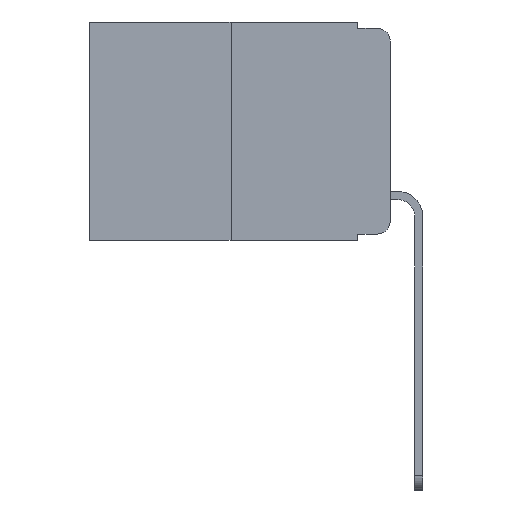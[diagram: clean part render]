
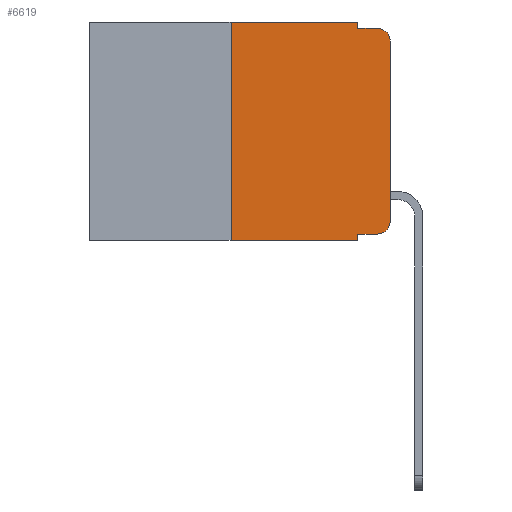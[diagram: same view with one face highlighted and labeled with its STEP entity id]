
A CAD part, left-side view. The second image highlights one B-rep face of the part: STEP entity #6619.
In plain terms, the highlighted planar face has unit normal (-1, 0, 0).
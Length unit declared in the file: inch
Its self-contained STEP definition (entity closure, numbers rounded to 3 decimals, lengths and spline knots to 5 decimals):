
#64 = DIRECTION ( 'NONE',  ( 0., 0., -1. ) ) ;
#298 = LINE ( 'NONE', #5664, #4951 ) ;
#318 = ORIENTED_EDGE ( 'NONE', *, *, #11865, .T. ) ;
#344 = VERTEX_POINT ( 'NONE', #5232 ) ;
#396 = LINE ( 'NONE', #3372, #3588 ) ;
#590 = CARTESIAN_POINT ( 'NONE',  ( 0., 0.02, -0.333 ) ) ;
#805 = CARTESIAN_POINT ( 'NONE',  ( 0., 0., -0.313 ) ) ;
#888 = EDGE_CURVE ( 'NONE', #10102, #5243, #298, .T. ) ;
#1156 = ORIENTED_EDGE ( 'NONE', *, *, #2356, .T. ) ;
#1325 = LINE ( 'NONE', #10715, #11564 ) ;
#1340 = VERTEX_POINT ( 'NONE', #6207 ) ;
#1586 = VECTOR ( 'NONE', #1956, 39.37008 ) ;
#1771 = DIRECTION ( 'NONE',  ( -1., 0., 0. ) ) ;
#1795 = CARTESIAN_POINT ( 'NONE',  ( 0., 0.02, -0.03 ) ) ;
#1818 = DIRECTION ( 'NONE',  ( 0., 0., 1. ) ) ;
#1942 = FACE_OUTER_BOUND ( 'NONE', #6504, .T. ) ;
#1956 = DIRECTION ( 'NONE',  ( 0., -1., 0. ) ) ;
#1960 = CARTESIAN_POINT ( 'NONE',  ( 0., 0.051, -0.01 ) ) ;
#2035 = CARTESIAN_POINT ( 'NONE',  ( 0., 0.473, 0. ) ) ;
#2044 = DIRECTION ( 'NONE',  ( 0., 0., -1. ) ) ;
#2119 = AXIS2_PLACEMENT_3D ( 'NONE', #1795, #1771, #2044 ) ;
#2172 = VERTEX_POINT ( 'NONE', #3794 ) ;
#2179 = EDGE_CURVE ( 'NONE', #2172, #10349, #2624, .T. ) ;
#2220 = PLANE ( 'NONE',  #6090 ) ;
#2356 = EDGE_CURVE ( 'NONE', #5243, #10670, #6807, .T. ) ;
#2624 = LINE ( 'NONE', #6823, #12651 ) ;
#2799 = CARTESIAN_POINT ( 'NONE',  ( 0., 0.02, -0.01 ) ) ;
#3025 = ORIENTED_EDGE ( 'NONE', *, *, #9255, .F. ) ;
#3040 = ORIENTED_EDGE ( 'NONE', *, *, #3772, .F. ) ;
#3073 = EDGE_CURVE ( 'NONE', #4557, #344, #396, .T. ) ;
#3372 = CARTESIAN_POINT ( 'NONE',  ( 0., 0.051, 0. ) ) ;
#3510 = ORIENTED_EDGE ( 'NONE', *, *, #2179, .T. ) ;
#3588 = VECTOR ( 'NONE', #10142, 39.37008 ) ;
#3754 = DIRECTION ( 'NONE',  ( 0., -1., 0. ) ) ;
#3772 = EDGE_CURVE ( 'NONE', #344, #10670, #6785, .T. ) ;
#3794 = CARTESIAN_POINT ( 'NONE',  ( 0., 0.25, -0.343 ) ) ;
#4047 = CIRCLE ( 'NONE', #5438, 0.02 ) ;
#4337 = ORIENTED_EDGE ( 'NONE', *, *, #6527, .F. ) ;
#4453 = VECTOR ( 'NONE', #11290, 39.37008 ) ;
#4557 = VERTEX_POINT ( 'NONE', #8699 ) ;
#4613 = VERTEX_POINT ( 'NONE', #11171 ) ;
#4899 = VECTOR ( 'NONE', #10902, 39.37008 ) ;
#4951 = VECTOR ( 'NONE', #9418, 39.37008 ) ;
#5050 = DIRECTION ( 'NONE',  ( -1., 0., 0. ) ) ;
#5150 = CARTESIAN_POINT ( 'NONE',  ( 0., 0.051, 0. ) ) ;
#5196 = DIRECTION ( 'NONE',  ( 0., -1., 0. ) ) ;
#5232 = CARTESIAN_POINT ( 'NONE',  ( 0., 0.051, -0.01 ) ) ;
#5243 = VERTEX_POINT ( 'NONE', #9652 ) ;
#5438 = AXIS2_PLACEMENT_3D ( 'NONE', #10813, #5050, #11738 ) ;
#5445 = ORIENTED_EDGE ( 'NONE', *, *, #6503, .F. ) ;
#5530 = CARTESIAN_POINT ( 'NONE',  ( 0., 0.051, -0.333 ) ) ;
#5542 = LINE ( 'NONE', #5150, #4899 ) ;
#5664 = CARTESIAN_POINT ( 'NONE',  ( 0., 0., 0. ) ) ;
#6090 = AXIS2_PLACEMENT_3D ( 'NONE', #9236, #6371, #64 ) ;
#6207 = CARTESIAN_POINT ( 'NONE',  ( 0., 0.051, -0.333 ) ) ;
#6320 = CARTESIAN_POINT ( 'NONE',  ( 0., 0.051, -0.343 ) ) ;
#6368 = VERTEX_POINT ( 'NONE', #590 ) ;
#6371 = DIRECTION ( 'NONE',  ( 1., 0., 0. ) ) ;
#6503 = EDGE_CURVE ( 'NONE', #1340, #10349, #5542, .T. ) ;
#6504 = EDGE_LOOP ( 'NONE', ( #9556, #1156, #3040, #12003, #4337, #3025, #3510, #5445, #318, #9163 ) ) ;
#6527 = EDGE_CURVE ( 'NONE', #4613, #4557, #7597, .T. ) ;
#6619 = ADVANCED_FACE ( 'NONE', ( #1942 ), #2220, .F. ) ;
#6785 = LINE ( 'NONE', #1960, #1586 ) ;
#6807 = CIRCLE ( 'NONE', #2119, 0.02 ) ;
#6823 = CARTESIAN_POINT ( 'NONE',  ( 0., 0.473, -0.343 ) ) ;
#7136 = LINE ( 'NONE', #5530, #4453 ) ;
#7597 = LINE ( 'NONE', #2035, #9477 ) ;
#8367 = EDGE_CURVE ( 'NONE', #6368, #10102, #4047, .T. ) ;
#8699 = CARTESIAN_POINT ( 'NONE',  ( 0., 0.051, 0. ) ) ;
#9163 = ORIENTED_EDGE ( 'NONE', *, *, #8367, .T. ) ;
#9236 = CARTESIAN_POINT ( 'NONE',  ( 0., 0.473, 0. ) ) ;
#9255 = EDGE_CURVE ( 'NONE', #2172, #4613, #1325, .T. ) ;
#9418 = DIRECTION ( 'NONE',  ( 0., 0., 1. ) ) ;
#9477 = VECTOR ( 'NONE', #5196, 39.37008 ) ;
#9556 = ORIENTED_EDGE ( 'NONE', *, *, #888, .T. ) ;
#9652 = CARTESIAN_POINT ( 'NONE',  ( 0., 0., -0.03 ) ) ;
#10102 = VERTEX_POINT ( 'NONE', #805 ) ;
#10142 = DIRECTION ( 'NONE',  ( 0., 0., -1. ) ) ;
#10349 = VERTEX_POINT ( 'NONE', #6320 ) ;
#10670 = VERTEX_POINT ( 'NONE', #2799 ) ;
#10715 = CARTESIAN_POINT ( 'NONE',  ( 0., 0.25, 0. ) ) ;
#10813 = CARTESIAN_POINT ( 'NONE',  ( 0., 0.02, -0.313 ) ) ;
#10902 = DIRECTION ( 'NONE',  ( 0., 0., -1. ) ) ;
#11171 = CARTESIAN_POINT ( 'NONE',  ( 0., 0.25, 0. ) ) ;
#11290 = DIRECTION ( 'NONE',  ( 0., -1., 0. ) ) ;
#11564 = VECTOR ( 'NONE', #1818, 39.37008 ) ;
#11738 = DIRECTION ( 'NONE',  ( 0., 0., -1. ) ) ;
#11865 = EDGE_CURVE ( 'NONE', #1340, #6368, #7136, .T. ) ;
#12003 = ORIENTED_EDGE ( 'NONE', *, *, #3073, .F. ) ;
#12651 = VECTOR ( 'NONE', #3754, 39.37008 ) ;
